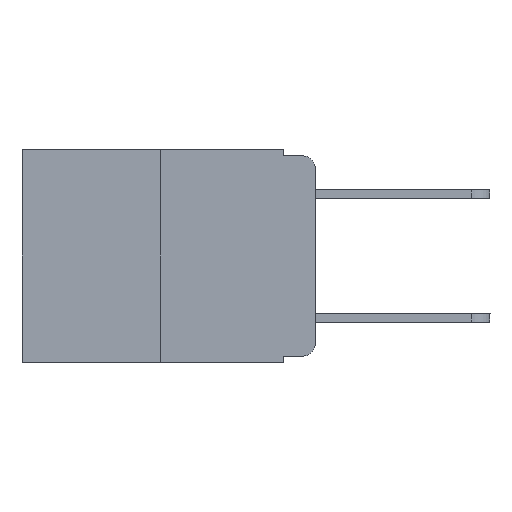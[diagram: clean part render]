
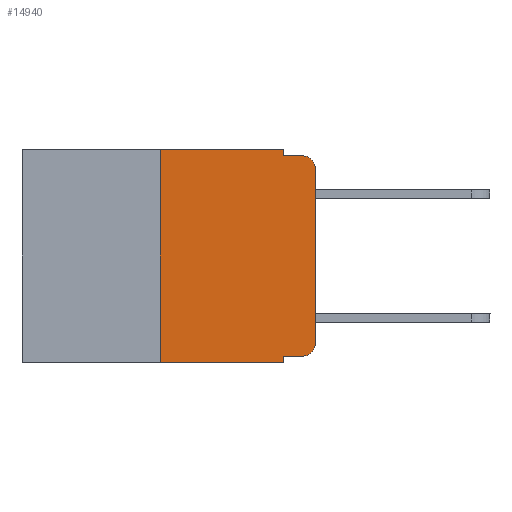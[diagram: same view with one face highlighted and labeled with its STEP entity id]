
A CAD part, left-side view. The second image highlights one B-rep face of the part: STEP entity #14940.
In plain terms, the highlighted planar face has unit normal (-1, 0, 0).
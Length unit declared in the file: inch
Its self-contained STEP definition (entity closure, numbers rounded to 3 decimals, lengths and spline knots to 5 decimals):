
#26 = VERTEX_POINT ( 'NONE', #9526 ) ;
#94 = CARTESIAN_POINT ( 'NONE',  ( 0., 0.051, 0. ) ) ;
#244 = DIRECTION ( 'NONE',  ( 1., 0., 0. ) ) ;
#356 = ORIENTED_EDGE ( 'NONE', *, *, #12483, .T. ) ;
#1104 = ORIENTED_EDGE ( 'NONE', *, *, #8868, .F. ) ;
#1325 = ORIENTED_EDGE ( 'NONE', *, *, #4320, .T. ) ;
#1580 = AXIS2_PLACEMENT_3D ( 'NONE', #4658, #11245, #6090 ) ;
#2092 = ORIENTED_EDGE ( 'NONE', *, *, #15079, .T. ) ;
#2233 = CARTESIAN_POINT ( 'NONE',  ( 0., 0.051, -0.333 ) ) ;
#2257 = CIRCLE ( 'NONE', #1580, 0.02 ) ;
#2395 = AXIS2_PLACEMENT_3D ( 'NONE', #10073, #16399, #15214 ) ;
#3092 = CARTESIAN_POINT ( 'NONE',  ( 0., 0.473, -0.343 ) ) ;
#3166 = CARTESIAN_POINT ( 'NONE',  ( 0., 0.25, -0.343 ) ) ;
#3323 = LINE ( 'NONE', #9561, #9352 ) ;
#3867 = VERTEX_POINT ( 'NONE', #11718 ) ;
#4257 = EDGE_LOOP ( 'NONE', ( #5203, #356, #8495, #1104, #6385, #9238, #2092, #15712, #6040, #1325 ) ) ;
#4309 = CARTESIAN_POINT ( 'NONE',  ( 0., 0.02, -0.01 ) ) ;
#4320 = EDGE_CURVE ( 'NONE', #9249, #3867, #2257, .T. ) ;
#4658 = CARTESIAN_POINT ( 'NONE',  ( 0., 0.02, -0.313 ) ) ;
#4826 = CARTESIAN_POINT ( 'NONE',  ( 0., 0.02, -0.333 ) ) ;
#5203 = ORIENTED_EDGE ( 'NONE', *, *, #9036, .T. ) ;
#5231 = CIRCLE ( 'NONE', #2395, 0.02 ) ;
#5257 = EDGE_CURVE ( 'NONE', #5613, #9249, #16112, .T. ) ;
#5303 = DIRECTION ( 'NONE',  ( 0., -1., 0. ) ) ;
#5337 = VERTEX_POINT ( 'NONE', #8632 ) ;
#5613 = VERTEX_POINT ( 'NONE', #15616 ) ;
#6040 = ORIENTED_EDGE ( 'NONE', *, *, #5257, .T. ) ;
#6090 = DIRECTION ( 'NONE',  ( 0., 0., -1. ) ) ;
#6324 = CARTESIAN_POINT ( 'NONE',  ( 0., 0.473, 0. ) ) ;
#6366 = CARTESIAN_POINT ( 'NONE',  ( 0., 0.051, -0.343 ) ) ;
#6385 = ORIENTED_EDGE ( 'NONE', *, *, #7208, .F. ) ;
#6533 = LINE ( 'NONE', #6324, #13990 ) ;
#6542 = DIRECTION ( 'NONE',  ( 0., 0., -1. ) ) ;
#6654 = LINE ( 'NONE', #94, #10680 ) ;
#7208 = EDGE_CURVE ( 'NONE', #7407, #12064, #6533, .T. ) ;
#7407 = VERTEX_POINT ( 'NONE', #10687 ) ;
#7682 = LINE ( 'NONE', #3092, #14140 ) ;
#8081 = FACE_OUTER_BOUND ( 'NONE', #4257, .T. ) ;
#8119 = DIRECTION ( 'NONE',  ( 0., 0., -1. ) ) ;
#8495 = ORIENTED_EDGE ( 'NONE', *, *, #14886, .F. ) ;
#8603 = CARTESIAN_POINT ( 'NONE',  ( 0., 0.25, 0. ) ) ;
#8632 = CARTESIAN_POINT ( 'NONE',  ( 0., 0., -0.03 ) ) ;
#8868 = EDGE_CURVE ( 'NONE', #12064, #26, #6654, .T. ) ;
#8941 = DIRECTION ( 'NONE',  ( 0., -1., 0. ) ) ;
#8989 = CARTESIAN_POINT ( 'NONE',  ( 0., 0.473, 0. ) ) ;
#9036 = EDGE_CURVE ( 'NONE', #3867, #5337, #15942, .T. ) ;
#9238 = ORIENTED_EDGE ( 'NONE', *, *, #9303, .F. ) ;
#9249 = VERTEX_POINT ( 'NONE', #4826 ) ;
#9303 = EDGE_CURVE ( 'NONE', #14133, #7407, #15725, .T. ) ;
#9352 = VECTOR ( 'NONE', #8119, 39.37008 ) ;
#9526 = CARTESIAN_POINT ( 'NONE',  ( 0., 0.051, -0.01 ) ) ;
#9561 = CARTESIAN_POINT ( 'NONE',  ( 0., 0.051, 0. ) ) ;
#10073 = CARTESIAN_POINT ( 'NONE',  ( 0., 0.02, -0.03 ) ) ;
#10484 = DIRECTION ( 'NONE',  ( 0., 0., 1. ) ) ;
#10493 = AXIS2_PLACEMENT_3D ( 'NONE', #8989, #244, #6542 ) ;
#10680 = VECTOR ( 'NONE', #14337, 39.37008 ) ;
#10687 = CARTESIAN_POINT ( 'NONE',  ( 0., 0.25, 0. ) ) ;
#11095 = VECTOR ( 'NONE', #12660, 39.37008 ) ;
#11245 = DIRECTION ( 'NONE',  ( -1., 0., 0. ) ) ;
#11669 = PLANE ( 'NONE',  #10493 ) ;
#11718 = CARTESIAN_POINT ( 'NONE',  ( 0., 0., -0.313 ) ) ;
#11825 = CARTESIAN_POINT ( 'NONE',  ( 0., 0.051, -0.01 ) ) ;
#12064 = VERTEX_POINT ( 'NONE', #15627 ) ;
#12158 = EDGE_CURVE ( 'NONE', #5613, #14332, #3323, .T. ) ;
#12483 = EDGE_CURVE ( 'NONE', #5337, #15819, #5231, .T. ) ;
#12660 = DIRECTION ( 'NONE',  ( 0., 0., 1. ) ) ;
#13239 = DIRECTION ( 'NONE',  ( 0., -1., 0. ) ) ;
#13990 = VECTOR ( 'NONE', #8941, 39.37008 ) ;
#13995 = DIRECTION ( 'NONE',  ( 0., -1., 0. ) ) ;
#14133 = VERTEX_POINT ( 'NONE', #3166 ) ;
#14140 = VECTOR ( 'NONE', #13239, 39.37008 ) ;
#14332 = VERTEX_POINT ( 'NONE', #6366 ) ;
#14336 = VECTOR ( 'NONE', #5303, 39.37008 ) ;
#14337 = DIRECTION ( 'NONE',  ( 0., 0., -1. ) ) ;
#14886 = EDGE_CURVE ( 'NONE', #26, #15819, #16348, .T. ) ;
#14940 = ADVANCED_FACE ( 'NONE', ( #8081 ), #11669, .F. ) ;
#15079 = EDGE_CURVE ( 'NONE', #14133, #14332, #7682, .T. ) ;
#15214 = DIRECTION ( 'NONE',  ( 0., 0., -1. ) ) ;
#15616 = CARTESIAN_POINT ( 'NONE',  ( 0., 0.051, -0.333 ) ) ;
#15627 = CARTESIAN_POINT ( 'NONE',  ( 0., 0.051, 0. ) ) ;
#15712 = ORIENTED_EDGE ( 'NONE', *, *, #12158, .F. ) ;
#15725 = LINE ( 'NONE', #8603, #11095 ) ;
#15734 = CARTESIAN_POINT ( 'NONE',  ( 0., 0., 0. ) ) ;
#15819 = VERTEX_POINT ( 'NONE', #4309 ) ;
#15896 = VECTOR ( 'NONE', #13995, 39.37008 ) ;
#15942 = LINE ( 'NONE', #15734, #16344 ) ;
#16112 = LINE ( 'NONE', #2233, #15896 ) ;
#16344 = VECTOR ( 'NONE', #10484, 39.37008 ) ;
#16348 = LINE ( 'NONE', #11825, #14336 ) ;
#16399 = DIRECTION ( 'NONE',  ( -1., 0., 0. ) ) ;
